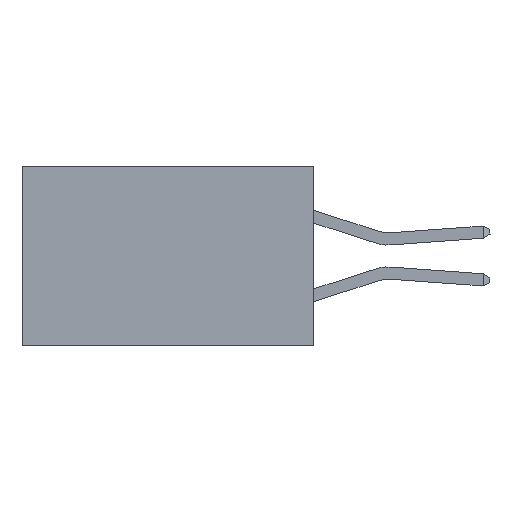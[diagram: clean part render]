
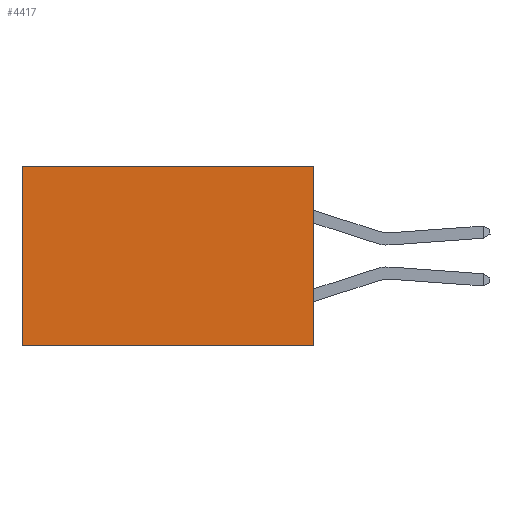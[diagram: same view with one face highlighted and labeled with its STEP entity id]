
A CAD part, left-side view. The second image highlights one B-rep face of the part: STEP entity #4417.
In plain terms, the highlighted planar face has unit normal (-1, 0, 0).
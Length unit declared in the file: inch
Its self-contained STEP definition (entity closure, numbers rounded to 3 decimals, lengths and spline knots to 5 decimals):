
#957 = CARTESIAN_POINT ( 'NONE',  ( 0.2875, 0., 0. ) ) ;
#1944 = CARTESIAN_POINT ( 'NONE',  ( 0.2875, 0., 0. ) ) ;
#1945 = EDGE_CURVE ( 'NONE', #5070, #4025, #2624, .T. ) ;
#2470 = CARTESIAN_POINT ( 'NONE',  ( 0.2875, 0.6, -0.37 ) ) ;
#2624 = LINE ( 'NONE', #4648, #4115 ) ;
#2768 = ORIENTED_EDGE ( 'NONE', *, *, #1945, .T. ) ;
#3387 = CARTESIAN_POINT ( 'NONE',  ( 0.2875, 0., 0. ) ) ;
#3545 = CARTESIAN_POINT ( 'NONE',  ( 0.2875, 0., -0.37 ) ) ;
#4025 = VERTEX_POINT ( 'NONE', #2470 ) ;
#4115 = VECTOR ( 'NONE', #9388, 39.37008 ) ;
#4389 = EDGE_CURVE ( 'NONE', #6378, #8031, #15078, .T. ) ;
#4417 = ADVANCED_FACE ( 'NONE', ( #10501 ), #7959, .F. ) ;
#4648 = CARTESIAN_POINT ( 'NONE',  ( 0.2875, 0.6, 0. ) ) ;
#5070 = VERTEX_POINT ( 'NONE', #15155 ) ;
#5639 = VECTOR ( 'NONE', #11990, 39.37008 ) ;
#6373 = EDGE_LOOP ( 'NONE', ( #2768, #7474, #13198, #10071 ) ) ;
#6378 = VERTEX_POINT ( 'NONE', #3387 ) ;
#7474 = ORIENTED_EDGE ( 'NONE', *, *, #13558, .F. ) ;
#7959 = PLANE ( 'NONE',  #8130 ) ;
#8031 = VERTEX_POINT ( 'NONE', #3545 ) ;
#8130 = AXIS2_PLACEMENT_3D ( 'NONE', #957, #15023, #14867 ) ;
#8616 = VECTOR ( 'NONE', #11960, 39.37008 ) ;
#9388 = DIRECTION ( 'NONE',  ( 0., 0., -1. ) ) ;
#9770 = CARTESIAN_POINT ( 'NONE',  ( 0.2875, 0., -0.37 ) ) ;
#10071 = ORIENTED_EDGE ( 'NONE', *, *, #10807, .T. ) ;
#10501 = FACE_OUTER_BOUND ( 'NONE', #6373, .T. ) ;
#10807 = EDGE_CURVE ( 'NONE', #6378, #5070, #13521, .T. ) ;
#10950 = CARTESIAN_POINT ( 'NONE',  ( 0.2875, 0., 0. ) ) ;
#11521 = LINE ( 'NONE', #9770, #5639 ) ;
#11937 = VECTOR ( 'NONE', #12600, 39.37008 ) ;
#11960 = DIRECTION ( 'NONE',  ( 0., 1., 0. ) ) ;
#11990 = DIRECTION ( 'NONE',  ( 0., 1., 0. ) ) ;
#12600 = DIRECTION ( 'NONE',  ( 0., 0., -1. ) ) ;
#13198 = ORIENTED_EDGE ( 'NONE', *, *, #4389, .F. ) ;
#13521 = LINE ( 'NONE', #10950, #8616 ) ;
#13558 = EDGE_CURVE ( 'NONE', #8031, #4025, #11521, .T. ) ;
#14867 = DIRECTION ( 'NONE',  ( 0., 0., -1. ) ) ;
#15023 = DIRECTION ( 'NONE',  ( 1., 0., 0. ) ) ;
#15078 = LINE ( 'NONE', #1944, #11937 ) ;
#15155 = CARTESIAN_POINT ( 'NONE',  ( 0.2875, 0.6, 0. ) ) ;
